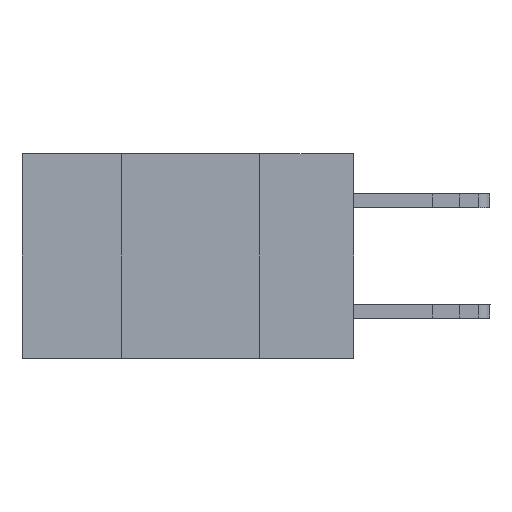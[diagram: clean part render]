
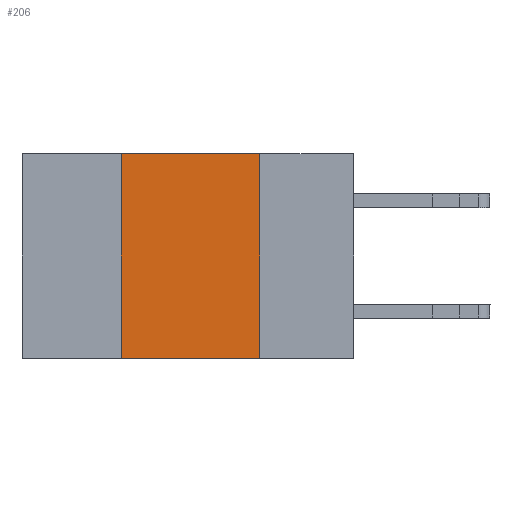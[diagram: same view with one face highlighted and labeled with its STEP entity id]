
A CAD part, left-side view. The second image highlights one B-rep face of the part: STEP entity #206.
In plain terms, the highlighted planar face has unit normal (-1, 0, 0).
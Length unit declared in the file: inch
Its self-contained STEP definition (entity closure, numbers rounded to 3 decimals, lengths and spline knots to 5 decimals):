
#206 = ADVANCED_FACE ( 'NONE', ( #6654 ), #2112, .F. ) ;
#392 = ORIENTED_EDGE ( 'NONE', *, *, #12279, .F. ) ;
#825 = EDGE_CURVE ( 'NONE', #3035, #19766, #4744, .T. ) ;
#1006 = DIRECTION ( 'NONE',  ( 0., -1., 0. ) ) ;
#2006 = LINE ( 'NONE', #16366, #22139 ) ;
#2112 = PLANE ( 'NONE',  #14437 ) ;
#2502 = CARTESIAN_POINT ( 'NONE',  ( 0., 0.6, 0. ) ) ;
#2718 = DIRECTION ( 'NONE',  ( 0., -1., 0. ) ) ;
#2960 = EDGE_CURVE ( 'NONE', #15670, #3035, #20388, .T. ) ;
#3035 = VERTEX_POINT ( 'NONE', #16379 ) ;
#3348 = CARTESIAN_POINT ( 'NONE',  ( 0., 0.17, -0.37 ) ) ;
#4383 = DIRECTION ( 'NONE',  ( 0., 0., -1. ) ) ;
#4744 = LINE ( 'NONE', #23117, #26473 ) ;
#4903 = ORIENTED_EDGE ( 'NONE', *, *, #825, .F. ) ;
#5479 = ORIENTED_EDGE ( 'NONE', *, *, #2960, .F. ) ;
#6654 = FACE_OUTER_BOUND ( 'NONE', #21193, .T. ) ;
#6658 = VECTOR ( 'NONE', #1006, 39.37008 ) ;
#6876 = CARTESIAN_POINT ( 'NONE',  ( 0., 0.42, -0.37 ) ) ;
#8073 = CARTESIAN_POINT ( 'NONE',  ( 0., 0.42, 0. ) ) ;
#11257 = LINE ( 'NONE', #19365, #6658 ) ;
#11828 = DIRECTION ( 'NONE',  ( 0., 0., 1. ) ) ;
#12279 = EDGE_CURVE ( 'NONE', #19766, #24575, #2006, .T. ) ;
#14437 = AXIS2_PLACEMENT_3D ( 'NONE', #2502, #18715, #4383 ) ;
#15670 = VERTEX_POINT ( 'NONE', #6876 ) ;
#16366 = CARTESIAN_POINT ( 'NONE',  ( 0., 0.17, 0. ) ) ;
#16379 = CARTESIAN_POINT ( 'NONE',  ( 0., 0.42, 0. ) ) ;
#18715 = DIRECTION ( 'NONE',  ( 1., 0., 0. ) ) ;
#19365 = CARTESIAN_POINT ( 'NONE',  ( 0., 0.6, -0.37 ) ) ;
#19766 = VERTEX_POINT ( 'NONE', #22359 ) ;
#19817 = DIRECTION ( 'NONE',  ( 0., 0., -1. ) ) ;
#20037 = VECTOR ( 'NONE', #11828, 39.37008 ) ;
#20388 = LINE ( 'NONE', #8073, #20037 ) ;
#20726 = ORIENTED_EDGE ( 'NONE', *, *, #23742, .T. ) ;
#21193 = EDGE_LOOP ( 'NONE', ( #392, #4903, #5479, #20726 ) ) ;
#22139 = VECTOR ( 'NONE', #19817, 39.37008 ) ;
#22359 = CARTESIAN_POINT ( 'NONE',  ( 0., 0.17, 0. ) ) ;
#23117 = CARTESIAN_POINT ( 'NONE',  ( 0., 0.6, 0. ) ) ;
#23742 = EDGE_CURVE ( 'NONE', #15670, #24575, #11257, .T. ) ;
#24575 = VERTEX_POINT ( 'NONE', #3348 ) ;
#26473 = VECTOR ( 'NONE', #2718, 39.37008 ) ;
